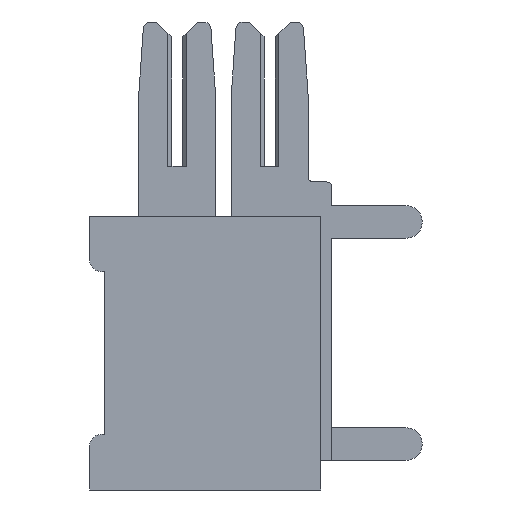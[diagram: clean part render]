
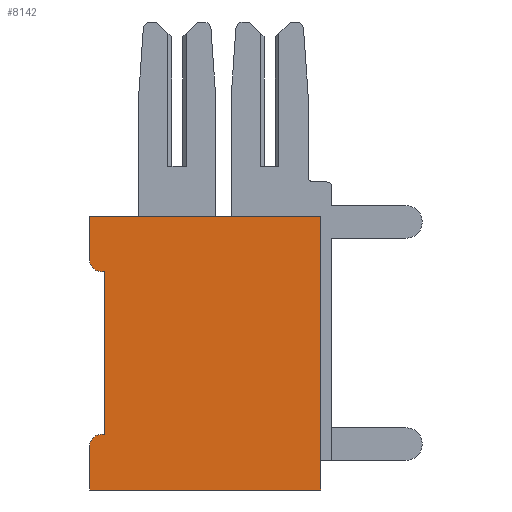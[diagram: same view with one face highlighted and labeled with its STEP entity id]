
A CAD part, left-side view. The second image highlights one B-rep face of the part: STEP entity #8142.
In plain terms, the highlighted planar face has unit normal (-1, 0, 0).
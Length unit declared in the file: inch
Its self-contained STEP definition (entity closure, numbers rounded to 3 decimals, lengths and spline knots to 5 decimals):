
#124 = VECTOR ( 'NONE', #6881, 39.37008 ) ;
#271 = EDGE_CURVE ( 'NONE', #4564, #2560, #5862, .T. ) ;
#383 = FACE_OUTER_BOUND ( 'NONE', #2759, .T. ) ;
#469 = CARTESIAN_POINT ( 'NONE',  ( 0., 0.312, -0.37 ) ) ;
#498 = LINE ( 'NONE', #3515, #5539 ) ;
#525 = ORIENTED_EDGE ( 'NONE', *, *, #993, .F. ) ;
#527 = VECTOR ( 'NONE', #6024, 39.37008 ) ;
#602 = CARTESIAN_POINT ( 'NONE',  ( 0., 0.292, -0.075 ) ) ;
#781 = ORIENTED_EDGE ( 'NONE', *, *, #8112, .F. ) ;
#792 = DIRECTION ( 'NONE',  ( -1., 0., 0. ) ) ;
#804 = VECTOR ( 'NONE', #6360, 39.37008 ) ;
#847 = LINE ( 'NONE', #4791, #8651 ) ;
#993 = EDGE_CURVE ( 'NONE', #4564, #7113, #2274, .T. ) ;
#1101 = EDGE_CURVE ( 'NONE', #2064, #7992, #6253, .T. ) ;
#1207 = CARTESIAN_POINT ( 'NONE',  ( 0., 0.292, -0.295 ) ) ;
#1441 = ORIENTED_EDGE ( 'NONE', *, *, #4106, .F. ) ;
#1512 = DIRECTION ( 'NONE',  ( 0., 0., 1. ) ) ;
#1693 = VERTEX_POINT ( 'NONE', #469 ) ;
#1714 = DIRECTION ( 'NONE',  ( 0., 0., 1. ) ) ;
#1796 = VERTEX_POINT ( 'NONE', #6992 ) ;
#1905 = CARTESIAN_POINT ( 'NONE',  ( 0., 0., 0. ) ) ;
#2064 = VERTEX_POINT ( 'NONE', #3144 ) ;
#2089 = PLANE ( 'NONE',  #4777 ) ;
#2274 = LINE ( 'NONE', #6943, #124 ) ;
#2345 = DIRECTION ( 'NONE',  ( -1., 0., 0. ) ) ;
#2348 = LINE ( 'NONE', #2518, #527 ) ;
#2377 = DIRECTION ( 'NONE',  ( 0., 0., 1. ) ) ;
#2447 = CARTESIAN_POINT ( 'NONE',  ( 0., 0.297, -0.06 ) ) ;
#2518 = CARTESIAN_POINT ( 'NONE',  ( 0., 0.312, -0.075 ) ) ;
#2560 = VERTEX_POINT ( 'NONE', #6744 ) ;
#2716 = LINE ( 'NONE', #1207, #3885 ) ;
#2759 = EDGE_LOOP ( 'NONE', ( #1441, #8742, #8415, #4157, #525, #8161, #6631, #3481, #5260, #781 ) ) ;
#3017 = VERTEX_POINT ( 'NONE', #602 ) ;
#3082 = VERTEX_POINT ( 'NONE', #3554 ) ;
#3144 = CARTESIAN_POINT ( 'NONE',  ( 0., 0., -0.37 ) ) ;
#3481 = ORIENTED_EDGE ( 'NONE', *, *, #6109, .T. ) ;
#3515 = CARTESIAN_POINT ( 'NONE',  ( 0., 0., 0. ) ) ;
#3554 = CARTESIAN_POINT ( 'NONE',  ( 0., 0.312, -0.06 ) ) ;
#3587 = CARTESIAN_POINT ( 'NONE',  ( 0., 0.297, -0.31 ) ) ;
#3781 = DIRECTION ( 'NONE',  ( -1., 0., 0. ) ) ;
#3832 = LINE ( 'NONE', #8168, #5894 ) ;
#3885 = VECTOR ( 'NONE', #8140, 39.37008 ) ;
#4106 = EDGE_CURVE ( 'NONE', #3082, #1796, #8105, .T. ) ;
#4157 = ORIENTED_EDGE ( 'NONE', *, *, #7150, .F. ) ;
#4194 = VERTEX_POINT ( 'NONE', #4860 ) ;
#4317 = AXIS2_PLACEMENT_3D ( 'NONE', #2447, #3781, #1714 ) ;
#4400 = VECTOR ( 'NONE', #6163, 39.37008 ) ;
#4451 = CARTESIAN_POINT ( 'NONE',  ( 0., 0.297, -0.295 ) ) ;
#4564 = VERTEX_POINT ( 'NONE', #4451 ) ;
#4777 = AXIS2_PLACEMENT_3D ( 'NONE', #6277, #792, #6910 ) ;
#4791 = CARTESIAN_POINT ( 'NONE',  ( 0., 0.312, -0.37 ) ) ;
#4852 = DIRECTION ( 'NONE',  ( 0., -1., 0. ) ) ;
#4860 = CARTESIAN_POINT ( 'NONE',  ( 0., 0.297, -0.075 ) ) ;
#5260 = ORIENTED_EDGE ( 'NONE', *, *, #1101, .T. ) ;
#5393 = AXIS2_PLACEMENT_3D ( 'NONE', #3587, #2345, #2377 ) ;
#5539 = VECTOR ( 'NONE', #4852, 39.37008 ) ;
#5862 = CIRCLE ( 'NONE', #5393, 0.015 ) ;
#5894 = VECTOR ( 'NONE', #7474, 39.37008 ) ;
#6016 = EDGE_CURVE ( 'NONE', #3017, #4194, #2348, .T. ) ;
#6024 = DIRECTION ( 'NONE',  ( 0., 1., 0. ) ) ;
#6084 = CARTESIAN_POINT ( 'NONE',  ( 0., 0.292, -0.295 ) ) ;
#6109 = EDGE_CURVE ( 'NONE', #1693, #2064, #3832, .T. ) ;
#6163 = DIRECTION ( 'NONE',  ( 0., 0., 1. ) ) ;
#6191 = CIRCLE ( 'NONE', #4317, 0.015 ) ;
#6253 = LINE ( 'NONE', #8260, #4400 ) ;
#6277 = CARTESIAN_POINT ( 'NONE',  ( 0., 0., -0.37 ) ) ;
#6322 = CARTESIAN_POINT ( 'NONE',  ( 0., 0.312, -0.37 ) ) ;
#6360 = DIRECTION ( 'NONE',  ( 0., 0., 1. ) ) ;
#6520 = EDGE_CURVE ( 'NONE', #1693, #2560, #847, .T. ) ;
#6631 = ORIENTED_EDGE ( 'NONE', *, *, #6520, .F. ) ;
#6744 = CARTESIAN_POINT ( 'NONE',  ( 0., 0.312, -0.31 ) ) ;
#6881 = DIRECTION ( 'NONE',  ( 0., -1., 0. ) ) ;
#6910 = DIRECTION ( 'NONE',  ( 0., 0., 1. ) ) ;
#6943 = CARTESIAN_POINT ( 'NONE',  ( 0., 0.312, -0.295 ) ) ;
#6992 = CARTESIAN_POINT ( 'NONE',  ( 0., 0.312, 0. ) ) ;
#7113 = VERTEX_POINT ( 'NONE', #6084 ) ;
#7150 = EDGE_CURVE ( 'NONE', #7113, #3017, #2716, .T. ) ;
#7474 = DIRECTION ( 'NONE',  ( 0., -1., 0. ) ) ;
#7992 = VERTEX_POINT ( 'NONE', #1905 ) ;
#8105 = LINE ( 'NONE', #6322, #804 ) ;
#8112 = EDGE_CURVE ( 'NONE', #1796, #7992, #498, .T. ) ;
#8140 = DIRECTION ( 'NONE',  ( 0., 0., 1. ) ) ;
#8142 = ADVANCED_FACE ( 'NONE', ( #383 ), #2089, .T. ) ;
#8161 = ORIENTED_EDGE ( 'NONE', *, *, #271, .T. ) ;
#8168 = CARTESIAN_POINT ( 'NONE',  ( 0., 0., -0.37 ) ) ;
#8260 = CARTESIAN_POINT ( 'NONE',  ( 0., 0., -0.37 ) ) ;
#8382 = EDGE_CURVE ( 'NONE', #3082, #4194, #6191, .T. ) ;
#8415 = ORIENTED_EDGE ( 'NONE', *, *, #6016, .F. ) ;
#8651 = VECTOR ( 'NONE', #1512, 39.37008 ) ;
#8742 = ORIENTED_EDGE ( 'NONE', *, *, #8382, .T. ) ;
